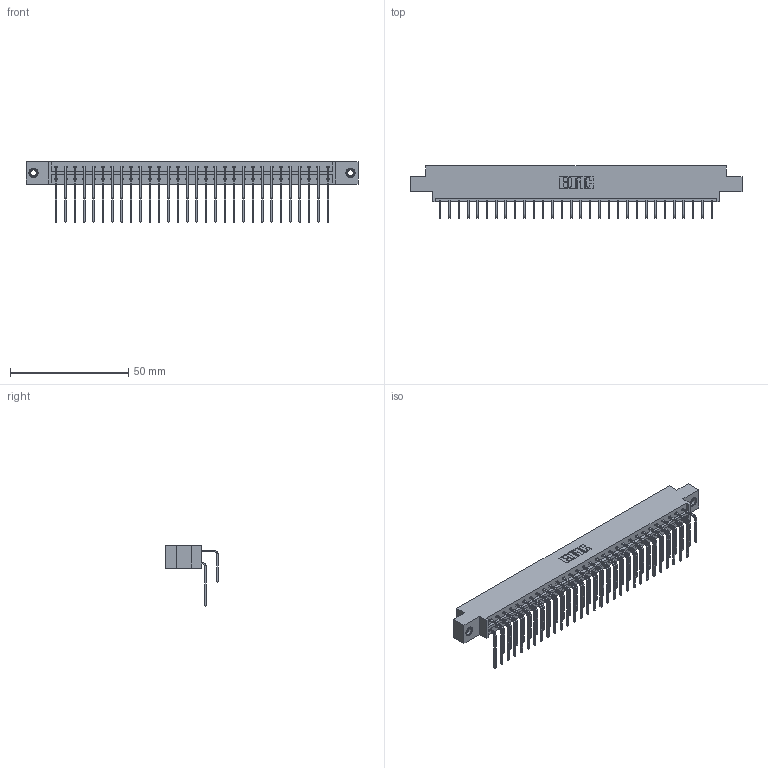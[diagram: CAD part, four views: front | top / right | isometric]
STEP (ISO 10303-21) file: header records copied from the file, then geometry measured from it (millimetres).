
FILE_DESCRIPTION (( 'STEP AP203' ), '1' );
FILE_NAME ('333-060-558-807.STEP', '2018-08-04T07:45:50', ( '' ), ( '' ), 'SwSTEP 2.0', 'SolidWorks 2016', '' );
FILE_SCHEMA (( 'CONFIG_CONTROL_DESIGN' ));
Length unit declared in the file: inch
Products named in the file (5): 345-292-001_558 559 Tail - 1; 345-292-001_558 Tail - 2; 345-250-001_345-250-005-103; 333-060-558-807; 333 Part_Offset - .156 Dia - TI
Assembly tree (63 placements, depth 2):
  333-060-558-807
    333 Part_Offset - .156 Dia - TI
    345-292-001_558 559 Tail - 1  x30
    345-292-001_558 Tail - 2  x30
    345-250-001_345-250-005-103  x2
Bounding box: 140.41 x 22.17 x 25.53 mm (x, y, z)
Volume: 14327.8 mm3; surface area: 18789.1 mm2
Topology: 63 solids, 63 shells, 3418 faces, 10119 edges, 6658 vertices
Faces by surface type: plane 2386, cylinder 1016, cone 12, torus 4
Entity records: 23954 total; most frequent: CARTESIAN_POINT 4020, ORIENTED_EDGE 3898, DIRECTION 3467, EDGE_CURVE 1949, VECTOR 1761, LINE 1761, VERTEX_POINT 1292, AXIS2_PLACEMENT_3D 853
